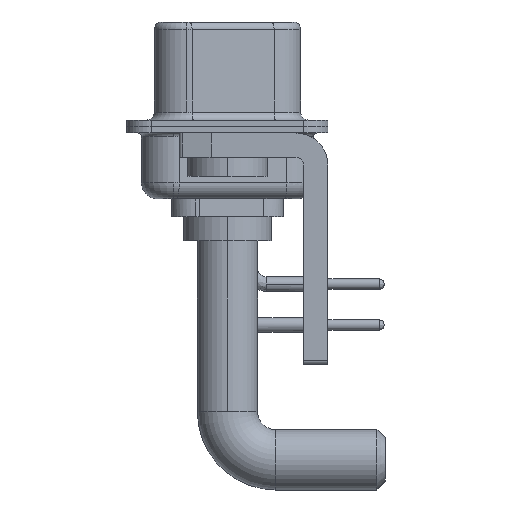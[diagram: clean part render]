
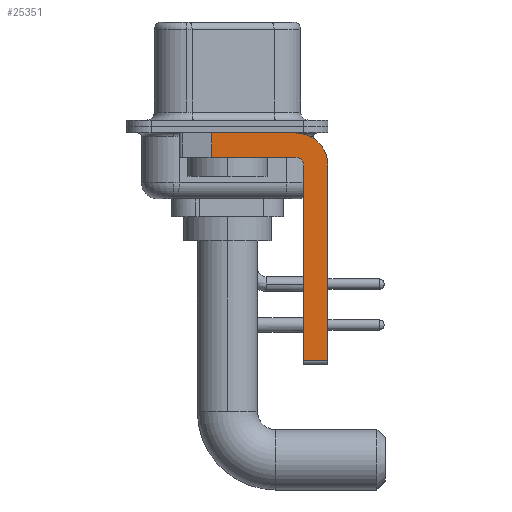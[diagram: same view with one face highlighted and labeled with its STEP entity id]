
A CAD part, left-side view. The second image highlights one B-rep face of the part: STEP entity #25351.
In plain terms, the highlighted planar face has unit normal (-1, 0, 0).
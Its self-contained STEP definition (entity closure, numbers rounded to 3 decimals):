
#205 = ORIENTED_EDGE ( 'NONE', *, *, #1721, .F. ) ;
#589 = VECTOR ( 'NONE', #11023, 1000. ) ;
#695 = VERTEX_POINT ( 'NONE', #1800 ) ;
#927 = ORIENTED_EDGE ( 'NONE', *, *, #1188, .F. ) ;
#1188 = EDGE_CURVE ( 'NONE', #9988, #1254, #13181, .T. ) ;
#1254 = VERTEX_POINT ( 'NONE', #11153 ) ;
#1659 = EDGE_CURVE ( 'NONE', #1254, #10812, #11366, .T. ) ;
#1685 = CARTESIAN_POINT ( 'NONE',  ( -2.9, -4.25, -1.9 ) ) ;
#1721 = EDGE_CURVE ( 'NONE', #21519, #15107, #26326, .T. ) ;
#1800 = CARTESIAN_POINT ( 'NONE',  ( -2.9, -6.25, -14.55 ) ) ;
#2439 = LINE ( 'NONE', #8505, #20262 ) ;
#2569 = DIRECTION ( 'NONE',  ( 0., -1., 0. ) ) ;
#3099 = ORIENTED_EDGE ( 'NONE', *, *, #7073, .T. ) ;
#3193 = AXIS2_PLACEMENT_3D ( 'NONE', #10740, #4952, #18963 ) ;
#3244 = ORIENTED_EDGE ( 'NONE', *, *, #15125, .F. ) ;
#4879 = AXIS2_PLACEMENT_3D ( 'NONE', #14898, #10320, #14632 ) ;
#4952 = DIRECTION ( 'NONE',  ( -1., 0., 0. ) ) ;
#5194 = CARTESIAN_POINT ( 'NONE',  ( -2.9, -4.75, -14.55 ) ) ;
#5653 = CARTESIAN_POINT ( 'NONE',  ( -2.9, 0.978, -0.4 ) ) ;
#6752 = VECTOR ( 'NONE', #17805, 1000. ) ;
#7073 = EDGE_CURVE ( 'NONE', #9988, #695, #2439, .T. ) ;
#7700 = DIRECTION ( 'NONE',  ( 0., 0., -1. ) ) ;
#8505 = CARTESIAN_POINT ( 'NONE',  ( -2.9, -4.25, -14.55 ) ) ;
#9808 = DIRECTION ( 'NONE',  ( 0., 0., -1. ) ) ;
#9851 = CARTESIAN_POINT ( 'NONE',  ( -2.9, -6.25, -2.4 ) ) ;
#9870 = AXIS2_PLACEMENT_3D ( 'NONE', #11881, #14294, #7700 ) ;
#9988 = VERTEX_POINT ( 'NONE', #5194 ) ;
#10320 = DIRECTION ( 'NONE',  ( 1., 0., 0. ) ) ;
#10640 = EDGE_CURVE ( 'NONE', #15107, #26569, #21198, .T. ) ;
#10740 = CARTESIAN_POINT ( 'NONE',  ( -2.9, -4.25, -2.4 ) ) ;
#10812 = VERTEX_POINT ( 'NONE', #21457 ) ;
#11023 = DIRECTION ( 'NONE',  ( 0., 0., 1. ) ) ;
#11153 = CARTESIAN_POINT ( 'NONE',  ( -2.9, -4.75, -2.4 ) ) ;
#11228 = ORIENTED_EDGE ( 'NONE', *, *, #1659, .F. ) ;
#11366 = CIRCLE ( 'NONE', #3193, 0.5 ) ;
#11796 = LINE ( 'NONE', #1685, #22226 ) ;
#11881 = CARTESIAN_POINT ( 'NONE',  ( -2.9, -4.25, -2.4 ) ) ;
#12694 = VECTOR ( 'NONE', #20024, 1000. ) ;
#13181 = LINE ( 'NONE', #17091, #589 ) ;
#13325 = VECTOR ( 'NONE', #9808, 1000. ) ;
#13988 = LINE ( 'NONE', #17896, #13325 ) ;
#14294 = DIRECTION ( 'NONE',  ( 1., 0., 0. ) ) ;
#14632 = DIRECTION ( 'NONE',  ( 0., 0., -1. ) ) ;
#14846 = EDGE_CURVE ( 'NONE', #26569, #695, #26382, .T. ) ;
#14898 = CARTESIAN_POINT ( 'NONE',  ( -2.9, -4.25, -2.4 ) ) ;
#14928 = VERTEX_POINT ( 'NONE', #24742 ) ;
#15107 = VERTEX_POINT ( 'NONE', #15420 ) ;
#15125 = EDGE_CURVE ( 'NONE', #10812, #14928, #11796, .T. ) ;
#15420 = CARTESIAN_POINT ( 'NONE',  ( -2.9, -4.25, -0.4 ) ) ;
#15862 = CARTESIAN_POINT ( 'NONE',  ( -2.9, 3., -0.4 ) ) ;
#17091 = CARTESIAN_POINT ( 'NONE',  ( -2.9, -4.75, -14.8 ) ) ;
#17805 = DIRECTION ( 'NONE',  ( 0., 0., -1. ) ) ;
#17896 = CARTESIAN_POINT ( 'NONE',  ( -2.9, 0.978, -1.9 ) ) ;
#18039 = ORIENTED_EDGE ( 'NONE', *, *, #10640, .F. ) ;
#18335 = ORIENTED_EDGE ( 'NONE', *, *, #14846, .F. ) ;
#18963 = DIRECTION ( 'NONE',  ( 0., 0., 1. ) ) ;
#19951 = FACE_OUTER_BOUND ( 'NONE', #24952, .T. ) ;
#20024 = DIRECTION ( 'NONE',  ( 0., -1., 0. ) ) ;
#20262 = VECTOR ( 'NONE', #2569, 1000. ) ;
#20297 = ORIENTED_EDGE ( 'NONE', *, *, #24533, .T. ) ;
#20460 = PLANE ( 'NONE',  #9870 ) ;
#21198 = CIRCLE ( 'NONE', #4879, 2. ) ;
#21457 = CARTESIAN_POINT ( 'NONE',  ( -2.9, -4.25, -1.9 ) ) ;
#21519 = VERTEX_POINT ( 'NONE', #5653 ) ;
#22226 = VECTOR ( 'NONE', #23997, 1000. ) ;
#23997 = DIRECTION ( 'NONE',  ( 0., 1., 0. ) ) ;
#24533 = EDGE_CURVE ( 'NONE', #21519, #14928, #13988, .T. ) ;
#24742 = CARTESIAN_POINT ( 'NONE',  ( -2.9, 0.978, -1.9 ) ) ;
#24952 = EDGE_LOOP ( 'NONE', ( #205, #20297, #3244, #11228, #927, #3099, #18335, #18039 ) ) ;
#25077 = CARTESIAN_POINT ( 'NONE',  ( -2.9, -6.25, -2.4 ) ) ;
#25351 = ADVANCED_FACE ( 'NONE', ( #19951 ), #20460, .F. ) ;
#26326 = LINE ( 'NONE', #15862, #12694 ) ;
#26382 = LINE ( 'NONE', #9851, #6752 ) ;
#26569 = VERTEX_POINT ( 'NONE', #25077 ) ;
